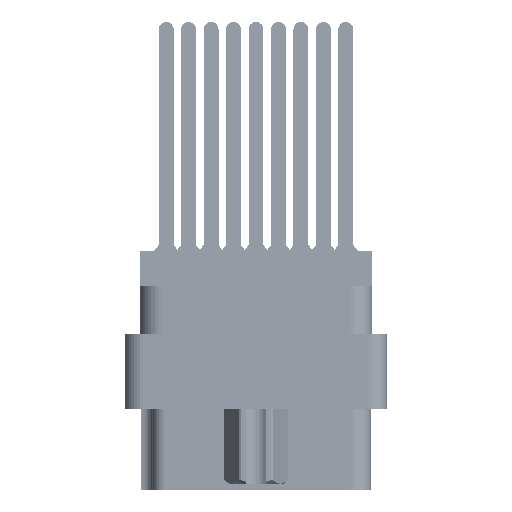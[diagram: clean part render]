
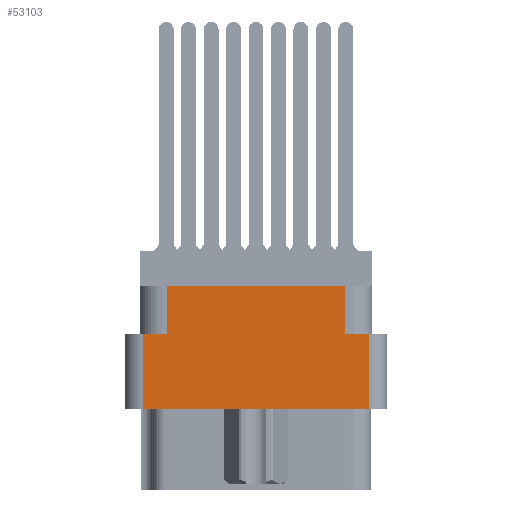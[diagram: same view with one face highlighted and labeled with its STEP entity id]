
A CAD part, left-side view. The second image highlights one B-rep face of the part: STEP entity #53103.
In plain terms, the highlighted planar face has unit normal (-1, 0, 0).
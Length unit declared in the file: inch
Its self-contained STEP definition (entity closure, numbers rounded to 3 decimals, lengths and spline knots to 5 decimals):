
#209 = CARTESIAN_POINT ( 'NONE',  ( -1.296, -0.376, -0.277 ) ) ;
#477 = CARTESIAN_POINT ( 'NONE',  ( -1.296, 0.296, -0.277 ) ) ;
#929 = VERTEX_POINT ( 'NONE', #52077 ) ;
#2089 = DIRECTION ( 'NONE',  ( 0., 1., 0. ) ) ;
#2560 = LINE ( 'NONE', #55902, #20619 ) ;
#2842 = LINE ( 'NONE', #28408, #14352 ) ;
#2955 = LINE ( 'NONE', #20655, #5150 ) ;
#3126 = PLANE ( 'NONE',  #40514 ) ;
#3990 = ORIENTED_EDGE ( 'NONE', *, *, #16843, .F. ) ;
#4890 = CARTESIAN_POINT ( 'NONE',  ( -1.296, 0.376, -0.798 ) ) ;
#5083 = EDGE_CURVE ( 'NONE', #929, #25541, #24027, .T. ) ;
#5150 = VECTOR ( 'NONE', #2089, 39.37008 ) ;
#6422 = EDGE_CURVE ( 'NONE', #54254, #51908, #35384, .T. ) ;
#6999 = VECTOR ( 'NONE', #37211, 39.37008 ) ;
#8553 = CARTESIAN_POINT ( 'NONE',  ( -1.296, -0.376, -0.529 ) ) ;
#9803 = DIRECTION ( 'NONE',  ( 0., 0., 1. ) ) ;
#11326 = DIRECTION ( 'NONE',  ( 0., -1., 0. ) ) ;
#14352 = VECTOR ( 'NONE', #24178, 39.37008 ) ;
#14727 = LINE ( 'NONE', #15765, #42991 ) ;
#15496 = CARTESIAN_POINT ( 'NONE',  ( -1.296, 0., -0.277 ) ) ;
#15765 = CARTESIAN_POINT ( 'NONE',  ( -1.296, 0., -0.277 ) ) ;
#15975 = EDGE_CURVE ( 'NONE', #51674, #20122, #27887, .T. ) ;
#16029 = EDGE_CURVE ( 'NONE', #56301, #51908, #2560, .T. ) ;
#16843 = EDGE_CURVE ( 'NONE', #54254, #20122, #14727, .T. ) ;
#17262 = CARTESIAN_POINT ( 'NONE',  ( -1.296, -0.296, -0.277 ) ) ;
#18509 = EDGE_CURVE ( 'NONE', #51674, #23731, #2955, .T. ) ;
#20122 = VERTEX_POINT ( 'NONE', #209 ) ;
#20619 = VECTOR ( 'NONE', #56502, 39.37008 ) ;
#20655 = CARTESIAN_POINT ( 'NONE',  ( -1.296, 0., -0.529 ) ) ;
#22448 = ORIENTED_EDGE ( 'NONE', *, *, #32429, .F. ) ;
#22709 = DIRECTION ( 'NONE',  ( 0., 0., 1. ) ) ;
#23731 = VERTEX_POINT ( 'NONE', #40397 ) ;
#24027 = LINE ( 'NONE', #15496, #29047 ) ;
#24178 = DIRECTION ( 'NONE',  ( 0., 0., 1. ) ) ;
#25541 = VERTEX_POINT ( 'NONE', #477 ) ;
#27392 = CARTESIAN_POINT ( 'NONE',  ( -1.296, 0.296, -0.117 ) ) ;
#27447 = VECTOR ( 'NONE', #40760, 39.37008 ) ;
#27887 = LINE ( 'NONE', #46261, #57526 ) ;
#28408 = CARTESIAN_POINT ( 'NONE',  ( -1.296, 0.296, -0.277 ) ) ;
#29047 = VECTOR ( 'NONE', #52880, 39.37008 ) ;
#29411 = ORIENTED_EDGE ( 'NONE', *, *, #18509, .F. ) ;
#32429 = EDGE_CURVE ( 'NONE', #25541, #56301, #2842, .T. ) ;
#33773 = LINE ( 'NONE', #4890, #6999 ) ;
#34016 = ORIENTED_EDGE ( 'NONE', *, *, #16029, .F. ) ;
#35384 = LINE ( 'NONE', #17262, #27447 ) ;
#36035 = DIRECTION ( 'NONE',  ( -1., 0., 0. ) ) ;
#36120 = FACE_OUTER_BOUND ( 'NONE', #54294, .T. ) ;
#37211 = DIRECTION ( 'NONE',  ( 0., 0., -1. ) ) ;
#39369 = ORIENTED_EDGE ( 'NONE', *, *, #15975, .T. ) ;
#40098 = CARTESIAN_POINT ( 'NONE',  ( -1.296, -0.438, -0.798 ) ) ;
#40397 = CARTESIAN_POINT ( 'NONE',  ( -1.296, 0.376, -0.529 ) ) ;
#40514 = AXIS2_PLACEMENT_3D ( 'NONE', #40098, #36035, #22709 ) ;
#40760 = DIRECTION ( 'NONE',  ( 0., 0., 1. ) ) ;
#40952 = ORIENTED_EDGE ( 'NONE', *, *, #55129, .T. ) ;
#41944 = CARTESIAN_POINT ( 'NONE',  ( -1.296, -0.296, -0.117 ) ) ;
#42991 = VECTOR ( 'NONE', #11326, 39.37008 ) ;
#45038 = ORIENTED_EDGE ( 'NONE', *, *, #6422, .T. ) ;
#45043 = CARTESIAN_POINT ( 'NONE',  ( -1.296, -0.296, -0.277 ) ) ;
#46261 = CARTESIAN_POINT ( 'NONE',  ( -1.296, -0.376, -0.798 ) ) ;
#51674 = VERTEX_POINT ( 'NONE', #8553 ) ;
#51908 = VERTEX_POINT ( 'NONE', #41944 ) ;
#52077 = CARTESIAN_POINT ( 'NONE',  ( -1.296, 0.376, -0.277 ) ) ;
#52880 = DIRECTION ( 'NONE',  ( 0., -1., 0. ) ) ;
#53103 = ADVANCED_FACE ( 'NONE', ( #36120 ), #3126, .T. ) ;
#54254 = VERTEX_POINT ( 'NONE', #45043 ) ;
#54294 = EDGE_LOOP ( 'NONE', ( #55984, #40952, #29411, #39369, #3990, #45038, #34016, #22448 ) ) ;
#55129 = EDGE_CURVE ( 'NONE', #929, #23731, #33773, .T. ) ;
#55902 = CARTESIAN_POINT ( 'NONE',  ( -1.296, 0.438, -0.117 ) ) ;
#55984 = ORIENTED_EDGE ( 'NONE', *, *, #5083, .F. ) ;
#56301 = VERTEX_POINT ( 'NONE', #27392 ) ;
#56502 = DIRECTION ( 'NONE',  ( 0., -1., 0. ) ) ;
#57526 = VECTOR ( 'NONE', #9803, 39.37008 ) ;
